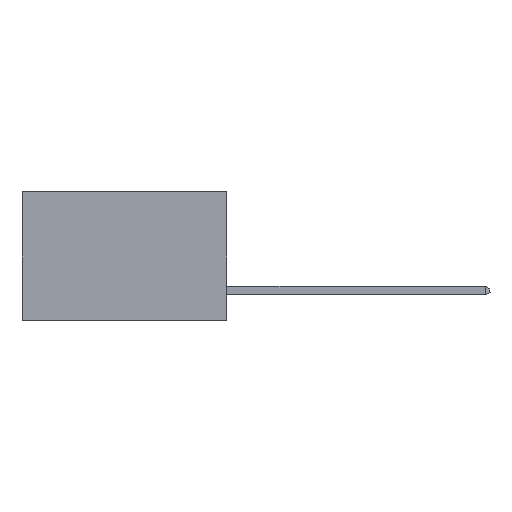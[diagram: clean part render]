
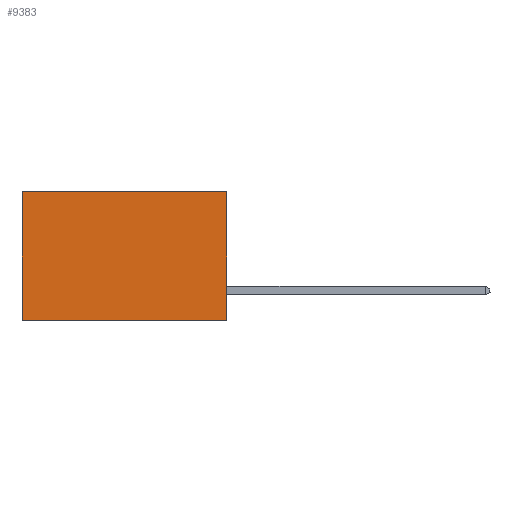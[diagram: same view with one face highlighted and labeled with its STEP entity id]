
A CAD part, left-side view. The second image highlights one B-rep face of the part: STEP entity #9383.
In plain terms, the highlighted planar face has unit normal (-1, 0, 0).
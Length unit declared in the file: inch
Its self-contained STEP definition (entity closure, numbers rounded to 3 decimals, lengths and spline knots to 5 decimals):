
#145 = CARTESIAN_POINT ( 'NONE',  ( 0.277, 0., 0. ) ) ;
#190 = EDGE_CURVE ( 'NONE', #15911, #20386, #10310, .T. ) ;
#3370 = DIRECTION ( 'NONE',  ( 0., 1., 0. ) ) ;
#3439 = VERTEX_POINT ( 'NONE', #9470 ) ;
#3444 = CARTESIAN_POINT ( 'NONE',  ( 0.277, 0., 0. ) ) ;
#3578 = VECTOR ( 'NONE', #18496, 39.37008 ) ;
#3936 = CARTESIAN_POINT ( 'NONE',  ( 0.277, 0., -0.37 ) ) ;
#4666 = LINE ( 'NONE', #15143, #3578 ) ;
#4825 = ORIENTED_EDGE ( 'NONE', *, *, #190, .F. ) ;
#5687 = DIRECTION ( 'NONE',  ( 0., 0., -1. ) ) ;
#5846 = CARTESIAN_POINT ( 'NONE',  ( 0.277, 0., -0.37 ) ) ;
#7039 = CARTESIAN_POINT ( 'NONE',  ( 0.277, 0., -0.37 ) ) ;
#7967 = EDGE_CURVE ( 'NONE', #15911, #13173, #17614, .T. ) ;
#9383 = ADVANCED_FACE ( 'NONE', ( #18298 ), #14142, .F. ) ;
#9470 = CARTESIAN_POINT ( 'NONE',  ( 0.277, 0.59, -0.37 ) ) ;
#10310 = LINE ( 'NONE', #5846, #18667 ) ;
#11359 = CARTESIAN_POINT ( 'NONE',  ( 0.277, 0., -0.37 ) ) ;
#11870 = AXIS2_PLACEMENT_3D ( 'NONE', #3936, #15821, #5687 ) ;
#11950 = DIRECTION ( 'NONE',  ( 0., 0., -1. ) ) ;
#13173 = VERTEX_POINT ( 'NONE', #21424 ) ;
#13952 = EDGE_CURVE ( 'NONE', #13173, #3439, #4666, .T. ) ;
#14142 = PLANE ( 'NONE',  #11870 ) ;
#15143 = CARTESIAN_POINT ( 'NONE',  ( 0.277, 0.59, -0.37 ) ) ;
#15821 = DIRECTION ( 'NONE',  ( 1., 0., 0. ) ) ;
#15911 = VERTEX_POINT ( 'NONE', #145 ) ;
#16365 = DIRECTION ( 'NONE',  ( 0., 1., 0. ) ) ;
#16579 = VECTOR ( 'NONE', #3370, 39.37008 ) ;
#16765 = EDGE_CURVE ( 'NONE', #20386, #3439, #17394, .T. ) ;
#17394 = LINE ( 'NONE', #11359, #20659 ) ;
#17412 = ORIENTED_EDGE ( 'NONE', *, *, #7967, .T. ) ;
#17614 = LINE ( 'NONE', #3444, #16579 ) ;
#18298 = FACE_OUTER_BOUND ( 'NONE', #20864, .T. ) ;
#18496 = DIRECTION ( 'NONE',  ( 0., 0., -1. ) ) ;
#18667 = VECTOR ( 'NONE', #11950, 39.37008 ) ;
#19227 = ORIENTED_EDGE ( 'NONE', *, *, #16765, .F. ) ;
#20386 = VERTEX_POINT ( 'NONE', #7039 ) ;
#20605 = ORIENTED_EDGE ( 'NONE', *, *, #13952, .T. ) ;
#20659 = VECTOR ( 'NONE', #16365, 39.37008 ) ;
#20864 = EDGE_LOOP ( 'NONE', ( #20605, #19227, #4825, #17412 ) ) ;
#21424 = CARTESIAN_POINT ( 'NONE',  ( 0.277, 0.59, 0. ) ) ;
